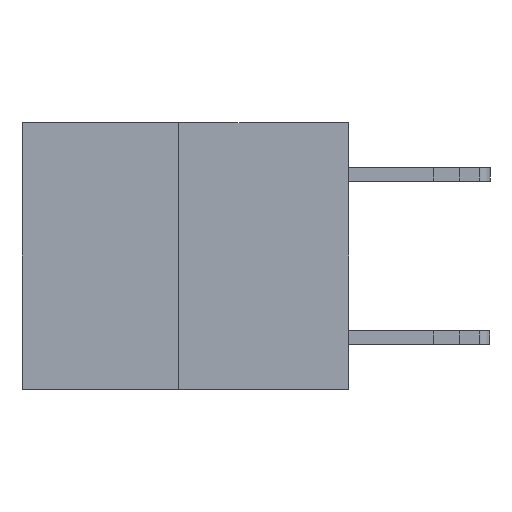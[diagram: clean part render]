
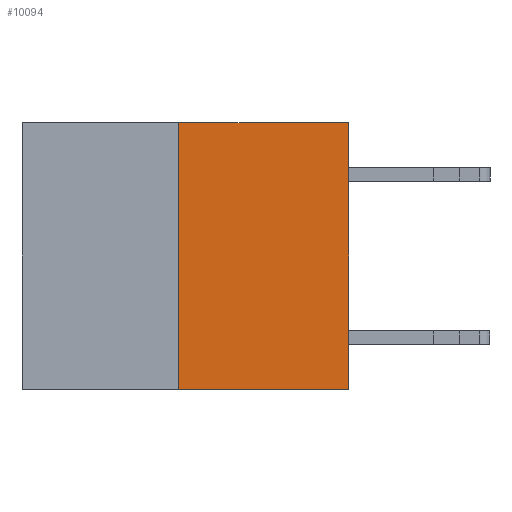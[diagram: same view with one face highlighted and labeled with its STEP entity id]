
A CAD part, left-side view. The second image highlights one B-rep face of the part: STEP entity #10094.
In plain terms, the highlighted planar face has unit normal (-1, 0, 0).
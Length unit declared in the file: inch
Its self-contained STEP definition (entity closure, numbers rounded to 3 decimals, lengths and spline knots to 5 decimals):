
#530 = ORIENTED_EDGE ( 'NONE', *, *, #5886, .F. ) ;
#640 = VECTOR ( 'NONE', #4066, 39.37008 ) ;
#2905 = DIRECTION ( 'NONE',  ( 0., 0., 1. ) ) ;
#3773 = LINE ( 'NONE', #19295, #7316 ) ;
#3797 = VECTOR ( 'NONE', #12028, 39.37008 ) ;
#4066 = DIRECTION ( 'NONE',  ( 0., 0., 1. ) ) ;
#4363 = PLANE ( 'NONE',  #5965 ) ;
#4768 = ORIENTED_EDGE ( 'NONE', *, *, #18799, .F. ) ;
#5808 = CARTESIAN_POINT ( 'NONE',  ( 0., 0., 0. ) ) ;
#5886 = EDGE_CURVE ( 'NONE', #9576, #17188, #3773, .T. ) ;
#5965 = AXIS2_PLACEMENT_3D ( 'NONE', #15696, #20846, #19343 ) ;
#7316 = VECTOR ( 'NONE', #2905, 39.37008 ) ;
#7323 = CARTESIAN_POINT ( 'NONE',  ( 0., 0.6, -0.49 ) ) ;
#7947 = CARTESIAN_POINT ( 'NONE',  ( 0., 0.6, 0. ) ) ;
#8757 = VERTEX_POINT ( 'NONE', #11171 ) ;
#8874 = LINE ( 'NONE', #7323, #3797 ) ;
#8989 = CARTESIAN_POINT ( 'NONE',  ( 0., 0., 0. ) ) ;
#9085 = LINE ( 'NONE', #7947, #9823 ) ;
#9576 = VERTEX_POINT ( 'NONE', #14906 ) ;
#9823 = VECTOR ( 'NONE', #16251, 39.37008 ) ;
#10094 = ADVANCED_FACE ( 'NONE', ( #12968 ), #4363, .F. ) ;
#11171 = CARTESIAN_POINT ( 'NONE',  ( 0., 0., -0.49 ) ) ;
#11292 = EDGE_CURVE ( 'NONE', #9576, #8757, #8874, .T. ) ;
#12028 = DIRECTION ( 'NONE',  ( 0., -1., 0. ) ) ;
#12889 = EDGE_CURVE ( 'NONE', #8757, #16332, #18110, .T. ) ;
#12968 = FACE_OUTER_BOUND ( 'NONE', #15124, .T. ) ;
#13136 = CARTESIAN_POINT ( 'NONE',  ( 0., 0.312, 0. ) ) ;
#13800 = ORIENTED_EDGE ( 'NONE', *, *, #12889, .T. ) ;
#14325 = ORIENTED_EDGE ( 'NONE', *, *, #11292, .T. ) ;
#14906 = CARTESIAN_POINT ( 'NONE',  ( 0., 0.312, -0.49 ) ) ;
#15124 = EDGE_LOOP ( 'NONE', ( #530, #14325, #13800, #4768 ) ) ;
#15696 = CARTESIAN_POINT ( 'NONE',  ( 0., 0.6, 0. ) ) ;
#16251 = DIRECTION ( 'NONE',  ( 0., -1., 0. ) ) ;
#16332 = VERTEX_POINT ( 'NONE', #5808 ) ;
#17188 = VERTEX_POINT ( 'NONE', #13136 ) ;
#18110 = LINE ( 'NONE', #8989, #640 ) ;
#18799 = EDGE_CURVE ( 'NONE', #17188, #16332, #9085, .T. ) ;
#19295 = CARTESIAN_POINT ( 'NONE',  ( 0., 0.312, -0.49 ) ) ;
#19343 = DIRECTION ( 'NONE',  ( 0., 0., -1. ) ) ;
#20846 = DIRECTION ( 'NONE',  ( 1., 0., 0. ) ) ;
